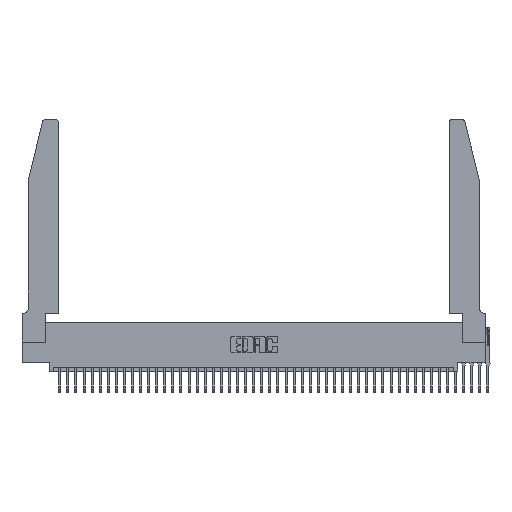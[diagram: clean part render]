
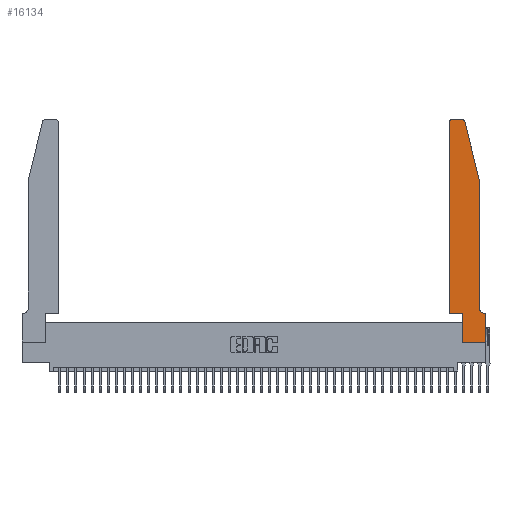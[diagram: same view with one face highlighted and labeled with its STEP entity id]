
A CAD part, top view. The second image highlights one B-rep face of the part: STEP entity #16134.
In plain terms, the highlighted face is planar.
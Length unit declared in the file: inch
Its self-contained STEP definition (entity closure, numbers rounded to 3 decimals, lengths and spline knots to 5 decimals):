
#69 = AXIS2_PLACEMENT_3D ( 'NONE', #20903, #1631, #24075 ) ;
#400 = ORIENTED_EDGE ( 'NONE', *, *, #31556, .T. ) ;
#620 = CARTESIAN_POINT ( 'NONE',  ( 0., 0., 0. ) ) ;
#1029 = EDGE_CURVE ( 'NONE', #31376, #34249, #38314, .T. ) ;
#1631 = DIRECTION ( 'NONE',  ( 0., 0., -1. ) ) ;
#1846 = CARTESIAN_POINT ( 'NONE',  ( 0., 0.35, 0. ) ) ;
#2563 = ORIENTED_EDGE ( 'NONE', *, *, #33058, .F. ) ;
#3018 = CIRCLE ( 'NONE', #5237, 0.03 ) ;
#3197 = CARTESIAN_POINT ( 'NONE',  ( 0.4505, 0.35, 0. ) ) ;
#3588 = EDGE_CURVE ( 'NONE', #3992, #4356, #9016, .T. ) ;
#3824 = ORIENTED_EDGE ( 'NONE', *, *, #24933, .T. ) ;
#3905 = DIRECTION ( 'NONE',  ( 1., 0., 0. ) ) ;
#3992 = VERTEX_POINT ( 'NONE', #40275 ) ;
#4356 = VERTEX_POINT ( 'NONE', #14078 ) ;
#4685 = DIRECTION ( 'NONE',  ( 0., -1., 0. ) ) ;
#5090 = DIRECTION ( 'NONE',  ( 0., 0., 1. ) ) ;
#5237 = AXIS2_PLACEMENT_3D ( 'NONE', #15725, #37646, #18916 ) ;
#7079 = CARTESIAN_POINT ( 'NONE',  ( 0.4505, 0.35, 0. ) ) ;
#7207 = CARTESIAN_POINT ( 'NONE',  ( 0.284, 2.75, 0. ) ) ;
#7824 = DIRECTION ( 'NONE',  ( 0., -1., 0. ) ) ;
#9016 = LINE ( 'NONE', #19431, #33271 ) ;
#9577 = CARTESIAN_POINT ( 'NONE',  ( 0.2605, 2.75, 0. ) ) ;
#9767 = ORIENTED_EDGE ( 'NONE', *, *, #3588, .F. ) ;
#9847 = ORIENTED_EDGE ( 'NONE', *, *, #38982, .F. ) ;
#10034 = EDGE_CURVE ( 'NONE', #34249, #23778, #26684, .T. ) ;
#10361 = DIRECTION ( 'NONE',  ( 0., 1., 0. ) ) ;
#11085 = VECTOR ( 'NONE', #21888, 39.37008 ) ;
#12240 = VERTEX_POINT ( 'NONE', #3197 ) ;
#12686 = CIRCLE ( 'NONE', #69, 0.07 ) ;
#13050 = VERTEX_POINT ( 'NONE', #7207 ) ;
#13411 = CARTESIAN_POINT ( 'NONE',  ( 0.0755, 0.35, 0. ) ) ;
#14078 = CARTESIAN_POINT ( 'NONE',  ( 0.0755, 2., 0. ) ) ;
#14319 = CARTESIAN_POINT ( 'NONE',  ( 0.4505, 2.72, 0. ) ) ;
#14684 = ORIENTED_EDGE ( 'NONE', *, *, #1029, .F. ) ;
#15340 = VERTEX_POINT ( 'NONE', #23777 ) ;
#15725 = CARTESIAN_POINT ( 'NONE',  ( 0.4205, 2.72, 0. ) ) ;
#15996 = LINE ( 'NONE', #620, #31771 ) ;
#16134 = ADVANCED_FACE ( 'NONE', ( #37867 ), #21096, .F. ) ;
#16275 = VECTOR ( 'NONE', #7824, 39.37008 ) ;
#16281 = LINE ( 'NONE', #17648, #23736 ) ;
#16473 = DIRECTION ( 'NONE',  ( -1., 0., 0. ) ) ;
#16508 = CARTESIAN_POINT ( 'NONE',  ( 0.2865, 0., 0. ) ) ;
#17309 = EDGE_CURVE ( 'NONE', #15340, #31376, #12686, .T. ) ;
#17648 = CARTESIAN_POINT ( 'NONE',  ( 0.0755, 2., 0. ) ) ;
#17832 = VERTEX_POINT ( 'NONE', #14319 ) ;
#18876 = CARTESIAN_POINT ( 'NONE',  ( 0.2865, 0.35, 0. ) ) ;
#18916 = DIRECTION ( 'NONE',  ( 1., 0., 0. ) ) ;
#19122 = CARTESIAN_POINT ( 'NONE',  ( 0.284, 2.72, 0. ) ) ;
#19146 = CARTESIAN_POINT ( 'NONE',  ( 0.0055, 0.35, 0. ) ) ;
#19431 = CARTESIAN_POINT ( 'NONE',  ( 0.0755, 2., 0. ) ) ;
#19704 = ORIENTED_EDGE ( 'NONE', *, *, #30223, .F. ) ;
#20065 = VERTEX_POINT ( 'NONE', #18876 ) ;
#20222 = LINE ( 'NONE', #25455, #27622 ) ;
#20903 = CARTESIAN_POINT ( 'NONE',  ( 0.0055, 0.42, 0. ) ) ;
#21096 = PLANE ( 'NONE',  #39372 ) ;
#21299 = AXIS2_PLACEMENT_3D ( 'NONE', #19122, #40952, #22314 ) ;
#21888 = DIRECTION ( 'NONE',  ( 1., 0., 0. ) ) ;
#22262 = VECTOR ( 'NONE', #10361, 39.37008 ) ;
#22314 = DIRECTION ( 'NONE',  ( 1., 0., 0. ) ) ;
#23654 = VECTOR ( 'NONE', #34842, 39.37008 ) ;
#23736 = VECTOR ( 'NONE', #4685, 39.37008 ) ;
#23763 = CARTESIAN_POINT ( 'NONE',  ( 0., 0., 0. ) ) ;
#23777 = CARTESIAN_POINT ( 'NONE',  ( 0.0755, 0.42, 0. ) ) ;
#23778 = VERTEX_POINT ( 'NONE', #25430 ) ;
#24075 = DIRECTION ( 'NONE',  ( -1., 0., 0. ) ) ;
#24206 = ORIENTED_EDGE ( 'NONE', *, *, #37377, .F. ) ;
#24933 = EDGE_CURVE ( 'NONE', #3992, #13050, #31738, .T. ) ;
#25430 = CARTESIAN_POINT ( 'NONE',  ( 0., 0., 0. ) ) ;
#25455 = CARTESIAN_POINT ( 'NONE',  ( 0.2865, 0.35, 0. ) ) ;
#25632 = LINE ( 'NONE', #9577, #23654 ) ;
#26684 = LINE ( 'NONE', #23763, #16275 ) ;
#27434 = DIRECTION ( 'NONE',  ( 1., 0., 0. ) ) ;
#27622 = VECTOR ( 'NONE', #34852, 39.37008 ) ;
#27826 = ORIENTED_EDGE ( 'NONE', *, *, #17309, .F. ) ;
#30223 = EDGE_CURVE ( 'NONE', #32254, #20065, #20222, .T. ) ;
#31376 = VERTEX_POINT ( 'NONE', #19146 ) ;
#31556 = EDGE_CURVE ( 'NONE', #33492, #17832, #3018, .T. ) ;
#31738 = CIRCLE ( 'NONE', #21299, 0.03 ) ;
#31771 = VECTOR ( 'NONE', #3905, 39.37008 ) ;
#31987 = CARTESIAN_POINT ( 'NONE',  ( 0.4205, 2.75, 0. ) ) ;
#32254 = VERTEX_POINT ( 'NONE', #16508 ) ;
#33058 = EDGE_CURVE ( 'NONE', #23778, #32254, #15996, .T. ) ;
#33271 = VECTOR ( 'NONE', #38139, 39.37008 ) ;
#33492 = VERTEX_POINT ( 'NONE', #31987 ) ;
#34249 = VERTEX_POINT ( 'NONE', #38374 ) ;
#34842 = DIRECTION ( 'NONE',  ( -1., 0., 0. ) ) ;
#34852 = DIRECTION ( 'NONE',  ( 0., 1., 0. ) ) ;
#35023 = ORIENTED_EDGE ( 'NONE', *, *, #36170, .F. ) ;
#35226 = LINE ( 'NONE', #40528, #11085 ) ;
#36170 = EDGE_CURVE ( 'NONE', #12240, #17832, #38820, .T. ) ;
#36363 = EDGE_CURVE ( 'NONE', #4356, #15340, #16281, .T. ) ;
#37377 = EDGE_CURVE ( 'NONE', #33492, #13050, #25632, .T. ) ;
#37646 = DIRECTION ( 'NONE',  ( 0., 0., -1. ) ) ;
#37867 = FACE_OUTER_BOUND ( 'NONE', #38695, .T. ) ;
#38139 = DIRECTION ( 'NONE',  ( -0.239, -0.971, 0. ) ) ;
#38314 = LINE ( 'NONE', #13411, #39286 ) ;
#38374 = CARTESIAN_POINT ( 'NONE',  ( 0., 0.35, 0. ) ) ;
#38695 = EDGE_LOOP ( 'NONE', ( #9767, #3824, #24206, #400, #35023, #9847, #19704, #2563, #39475, #14684, #27826, #40245 ) ) ;
#38820 = LINE ( 'NONE', #7079, #22262 ) ;
#38982 = EDGE_CURVE ( 'NONE', #20065, #12240, #35226, .T. ) ;
#39286 = VECTOR ( 'NONE', #16473, 39.37008 ) ;
#39372 = AXIS2_PLACEMENT_3D ( 'NONE', #1846, #5090, #27434 ) ;
#39475 = ORIENTED_EDGE ( 'NONE', *, *, #10034, .F. ) ;
#40245 = ORIENTED_EDGE ( 'NONE', *, *, #36363, .F. ) ;
#40275 = CARTESIAN_POINT ( 'NONE',  ( 0.25487, 2.72718, 0. ) ) ;
#40528 = CARTESIAN_POINT ( 'NONE',  ( 0.4505, 0.35, 0. ) ) ;
#40952 = DIRECTION ( 'NONE',  ( 0., 0., -1. ) ) ;
